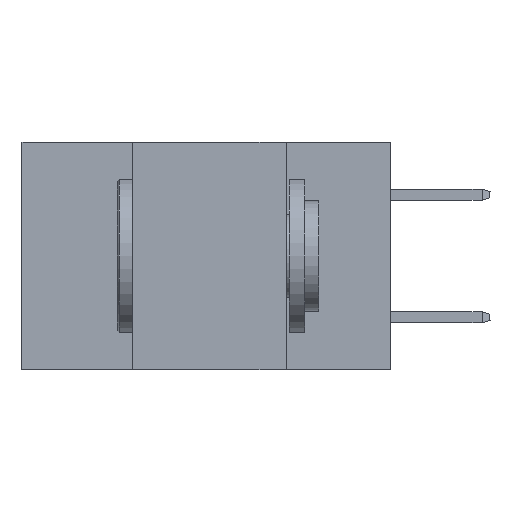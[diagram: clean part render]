
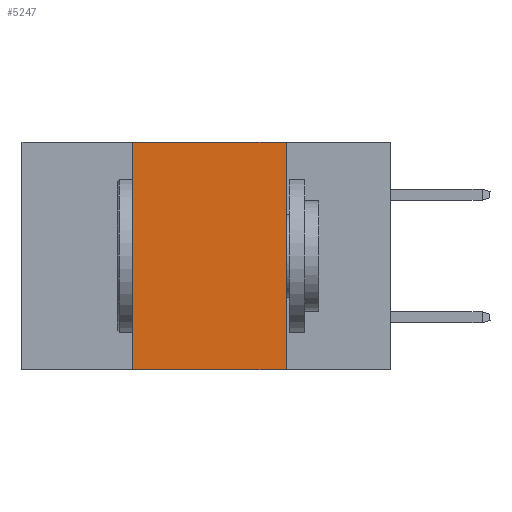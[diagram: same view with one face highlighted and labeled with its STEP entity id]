
A CAD part, left-side view. The second image highlights one B-rep face of the part: STEP entity #5247.
In plain terms, the highlighted planar face has unit normal (-1, 0, 0).
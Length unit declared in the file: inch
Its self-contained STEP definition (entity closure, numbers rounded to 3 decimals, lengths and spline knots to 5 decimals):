
#1760 = ORIENTED_EDGE ( 'NONE', *, *, #24247, .F. ) ;
#1969 = CARTESIAN_POINT ( 'NONE',  ( 0., 0.42, -0.37 ) ) ;
#4224 = EDGE_LOOP ( 'NONE', ( #1760, #34278, #25510, #15585 ) ) ;
#4444 = EDGE_CURVE ( 'NONE', #7307, #23570, #10616, .T. ) ;
#5247 = ADVANCED_FACE ( 'NONE', ( #23766 ), #21480, .F. ) ;
#6634 = CARTESIAN_POINT ( 'NONE',  ( 0., 0.6, 0. ) ) ;
#7307 = VERTEX_POINT ( 'NONE', #33272 ) ;
#8216 = VERTEX_POINT ( 'NONE', #22061 ) ;
#10616 = LINE ( 'NONE', #6634, #13802 ) ;
#12010 = VECTOR ( 'NONE', #19533, 39.37008 ) ;
#12106 = DIRECTION ( 'NONE',  ( 0., -1., 0. ) ) ;
#12919 = CARTESIAN_POINT ( 'NONE',  ( 0., 0.6, 0. ) ) ;
#13249 = VECTOR ( 'NONE', #21977, 39.37008 ) ;
#13802 = VECTOR ( 'NONE', #21140, 39.37008 ) ;
#15585 = ORIENTED_EDGE ( 'NONE', *, *, #29098, .T. ) ;
#15866 = DIRECTION ( 'NONE',  ( 1., 0., 0. ) ) ;
#16957 = CARTESIAN_POINT ( 'NONE',  ( 0., 0.17, 0. ) ) ;
#17974 = AXIS2_PLACEMENT_3D ( 'NONE', #12919, #15866, #36271 ) ;
#19533 = DIRECTION ( 'NONE',  ( 0., 0., -1. ) ) ;
#21140 = DIRECTION ( 'NONE',  ( 0., -1., 0. ) ) ;
#21480 = PLANE ( 'NONE',  #17974 ) ;
#21977 = DIRECTION ( 'NONE',  ( 0., 0., 1. ) ) ;
#22061 = CARTESIAN_POINT ( 'NONE',  ( 0., 0.17, -0.37 ) ) ;
#22918 = VERTEX_POINT ( 'NONE', #1969 ) ;
#23570 = VERTEX_POINT ( 'NONE', #16957 ) ;
#23766 = FACE_OUTER_BOUND ( 'NONE', #4224, .T. ) ;
#24247 = EDGE_CURVE ( 'NONE', #23570, #8216, #29411, .T. ) ;
#24382 = CARTESIAN_POINT ( 'NONE',  ( 0., 0.42, 0. ) ) ;
#25510 = ORIENTED_EDGE ( 'NONE', *, *, #34064, .F. ) ;
#26541 = LINE ( 'NONE', #24382, #13249 ) ;
#26896 = VECTOR ( 'NONE', #12106, 39.37008 ) ;
#29098 = EDGE_CURVE ( 'NONE', #22918, #8216, #35063, .T. ) ;
#29411 = LINE ( 'NONE', #31120, #12010 ) ;
#29621 = CARTESIAN_POINT ( 'NONE',  ( 0., 0.6, -0.37 ) ) ;
#31120 = CARTESIAN_POINT ( 'NONE',  ( 0., 0.17, 0. ) ) ;
#33272 = CARTESIAN_POINT ( 'NONE',  ( 0., 0.42, 0. ) ) ;
#34064 = EDGE_CURVE ( 'NONE', #22918, #7307, #26541, .T. ) ;
#34278 = ORIENTED_EDGE ( 'NONE', *, *, #4444, .F. ) ;
#35063 = LINE ( 'NONE', #29621, #26896 ) ;
#36271 = DIRECTION ( 'NONE',  ( 0., 0., -1. ) ) ;
